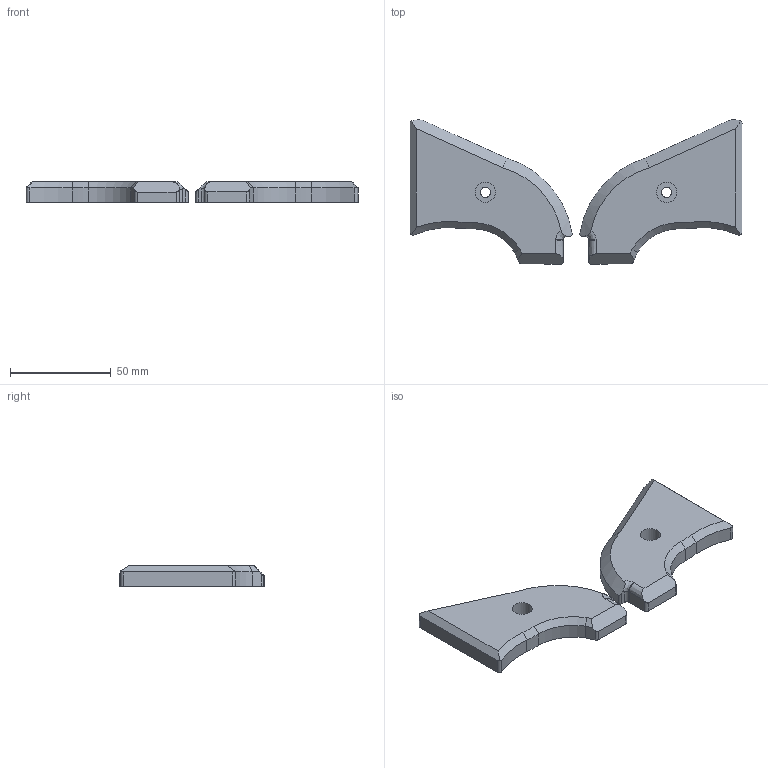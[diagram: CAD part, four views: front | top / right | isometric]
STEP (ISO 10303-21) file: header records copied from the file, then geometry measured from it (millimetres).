
FILE_DESCRIPTION(/* description */ (''),/* implementation_level */ '2;1');
FILE_NAME(/* name */ 'HRR - Plain Grips v3.step',/* time_stamp */ '2019-12-25T01:11:00-05:00',/* author */ (''),/* organization */ (''),/* preprocessor_version */ 'ST-DEVELOPER v18',/* originating_system */ 'Autodesk Translation Framework v8.12.0.6',/* authorisation */ '');
FILE_SCHEMA (('AUTOMOTIVE_DESIGN { 1 0 10303 214 3 1 1 }'));
Length unit declared in the file: inch
Products named in the file (1): HRR - Plain Grips
Bounding box: 164.75 x 71.66 x 10.19 mm (x, y, z)
Volume: 64761.2 mm3; surface area: 18522.3 mm2
Topology: 2 solids, 2 shells, 72 faces, 184 edges, 120 vertices
Faces by surface type: plane 30, cylinder 28, cone 8, bspline 6
Full cylindrical faces by diameter (mm): 4.39 x2, 5 x2, 10 x1, 10.075 x1
Entity records: 2596 total; most frequent: CARTESIAN_POINT 833, ORIENTED_EDGE 368, DIRECTION 350, EDGE_CURVE 184, AXIS2_PLACEMENT_3D 133, VERTEX_POINT 120, LINE 84, VECTOR 84
